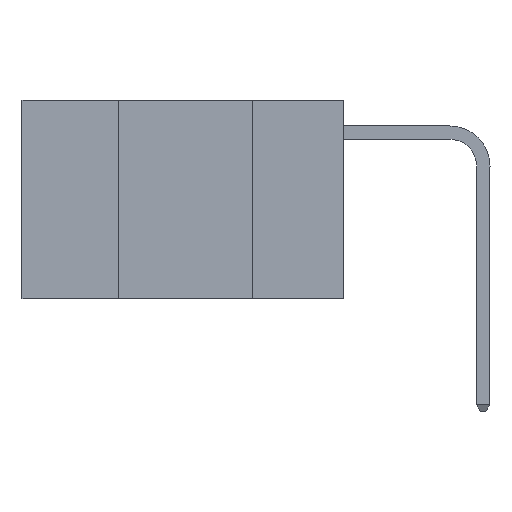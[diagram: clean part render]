
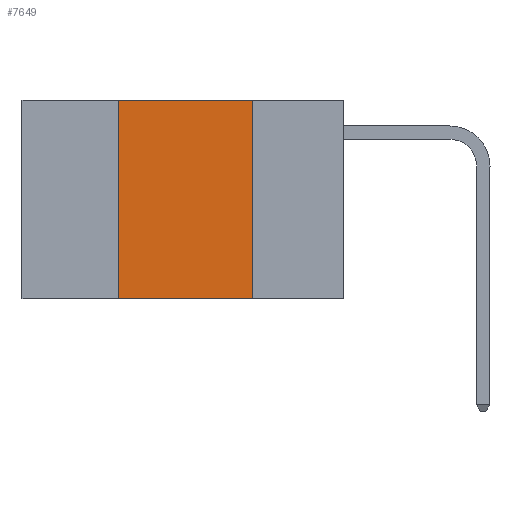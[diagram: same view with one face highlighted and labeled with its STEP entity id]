
A CAD part, left-side view. The second image highlights one B-rep face of the part: STEP entity #7649.
In plain terms, the highlighted planar face has unit normal (-1, 0, 0).
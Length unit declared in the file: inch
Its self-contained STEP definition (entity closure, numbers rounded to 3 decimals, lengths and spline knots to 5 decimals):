
#208 = CARTESIAN_POINT ( 'NONE',  ( 0., 0.42, -0.37 ) ) ;
#573 = CARTESIAN_POINT ( 'NONE',  ( 0., 0.17, 0. ) ) ;
#774 = PLANE ( 'NONE',  #10054 ) ;
#857 = LINE ( 'NONE', #4436, #3466 ) ;
#1669 = CARTESIAN_POINT ( 'NONE',  ( 0., 0.17, 0. ) ) ;
#1752 = VECTOR ( 'NONE', #6428, 39.37008 ) ;
#1894 = DIRECTION ( 'NONE',  ( 0., 0., -1. ) ) ;
#3030 = ORIENTED_EDGE ( 'NONE', *, *, #10674, .T. ) ;
#3466 = VECTOR ( 'NONE', #12898, 39.37008 ) ;
#3914 = DIRECTION ( 'NONE',  ( 0., 0., -1. ) ) ;
#4039 = CARTESIAN_POINT ( 'NONE',  ( 0., 0.6, 0. ) ) ;
#4050 = VERTEX_POINT ( 'NONE', #208 ) ;
#4356 = ORIENTED_EDGE ( 'NONE', *, *, #9212, .F. ) ;
#4436 = CARTESIAN_POINT ( 'NONE',  ( 0., 0.6, -0.37 ) ) ;
#5884 = DIRECTION ( 'NONE',  ( 0., 0., 1. ) ) ;
#6176 = LINE ( 'NONE', #573, #8633 ) ;
#6428 = DIRECTION ( 'NONE',  ( 0., -1., 0. ) ) ;
#7649 = ADVANCED_FACE ( 'NONE', ( #9138 ), #774, .F. ) ;
#7696 = VERTEX_POINT ( 'NONE', #9401 ) ;
#8303 = DIRECTION ( 'NONE',  ( 1., 0., 0. ) ) ;
#8633 = VECTOR ( 'NONE', #3914, 39.37008 ) ;
#9138 = FACE_OUTER_BOUND ( 'NONE', #12907, .T. ) ;
#9153 = EDGE_CURVE ( 'NONE', #4050, #9449, #12452, .T. ) ;
#9212 = EDGE_CURVE ( 'NONE', #11019, #7696, #6176, .T. ) ;
#9401 = CARTESIAN_POINT ( 'NONE',  ( 0., 0.17, -0.37 ) ) ;
#9449 = VERTEX_POINT ( 'NONE', #12843 ) ;
#9876 = EDGE_CURVE ( 'NONE', #9449, #11019, #10283, .T. ) ;
#10054 = AXIS2_PLACEMENT_3D ( 'NONE', #4039, #8303, #1894 ) ;
#10278 = ORIENTED_EDGE ( 'NONE', *, *, #9153, .F. ) ;
#10283 = LINE ( 'NONE', #11668, #1752 ) ;
#10285 = ORIENTED_EDGE ( 'NONE', *, *, #9876, .F. ) ;
#10674 = EDGE_CURVE ( 'NONE', #4050, #7696, #857, .T. ) ;
#11019 = VERTEX_POINT ( 'NONE', #1669 ) ;
#11187 = CARTESIAN_POINT ( 'NONE',  ( 0., 0.42, 0. ) ) ;
#11668 = CARTESIAN_POINT ( 'NONE',  ( 0., 0.6, 0. ) ) ;
#12117 = VECTOR ( 'NONE', #5884, 39.37008 ) ;
#12452 = LINE ( 'NONE', #11187, #12117 ) ;
#12843 = CARTESIAN_POINT ( 'NONE',  ( 0., 0.42, 0. ) ) ;
#12898 = DIRECTION ( 'NONE',  ( 0., -1., 0. ) ) ;
#12907 = EDGE_LOOP ( 'NONE', ( #4356, #10285, #10278, #3030 ) ) ;
